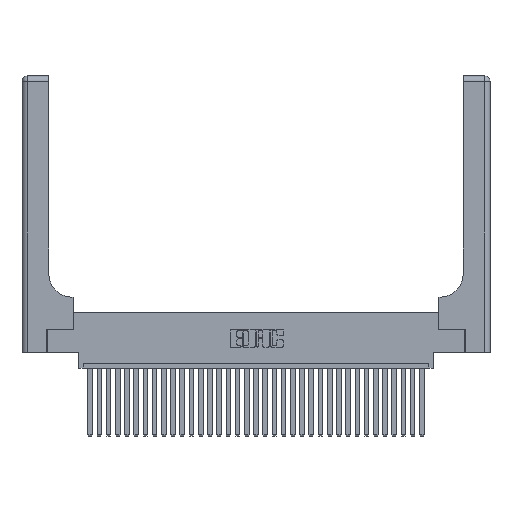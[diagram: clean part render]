
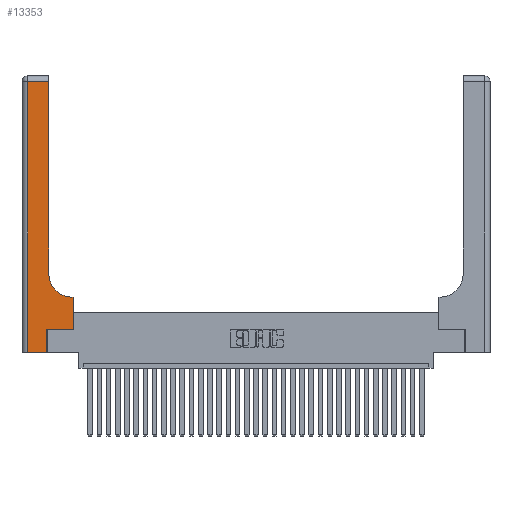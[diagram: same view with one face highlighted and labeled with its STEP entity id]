
A CAD part, top view. The second image highlights one B-rep face of the part: STEP entity #13353.
In plain terms, the highlighted planar face has unit normal (0, 0, 1).
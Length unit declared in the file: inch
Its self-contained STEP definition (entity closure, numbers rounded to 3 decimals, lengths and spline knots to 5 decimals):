
#236 = VERTEX_POINT ( 'NONE', #25386 ) ;
#242 = CARTESIAN_POINT ( 'NONE',  ( 0., 2.94, 0.37 ) ) ;
#461 = CARTESIAN_POINT ( 'NONE',  ( 0.269, 0.25, 0.37 ) ) ;
#1861 = VECTOR ( 'NONE', #8779, 39.37008 ) ;
#2887 = ORIENTED_EDGE ( 'NONE', *, *, #11937, .T. ) ;
#3539 = CARTESIAN_POINT ( 'NONE',  ( 0.2915, 3., 0.37 ) ) ;
#4384 = VERTEX_POINT ( 'NONE', #17243 ) ;
#4516 = DIRECTION ( 'NONE',  ( -1., 0., 0. ) ) ;
#4655 = ORIENTED_EDGE ( 'NONE', *, *, #23702, .T. ) ;
#5035 = LINE ( 'NONE', #22407, #10288 ) ;
#6044 = LINE ( 'NONE', #19729, #22750 ) ;
#6705 = EDGE_CURVE ( 'NONE', #28600, #26477, #22042, .T. ) ;
#6734 = ORIENTED_EDGE ( 'NONE', *, *, #29484, .T. ) ;
#7010 = ORIENTED_EDGE ( 'NONE', *, *, #10137, .T. ) ;
#7316 = CARTESIAN_POINT ( 'NONE',  ( 0., 0., 0.37 ) ) ;
#8605 = VERTEX_POINT ( 'NONE', #30904 ) ;
#8779 = DIRECTION ( 'NONE',  ( 1., 0., 0. ) ) ;
#9307 = VERTEX_POINT ( 'NONE', #14471 ) ;
#9494 = PLANE ( 'NONE',  #14238 ) ;
#9602 = CARTESIAN_POINT ( 'NONE',  ( 0.2915, 0.85, 0.37 ) ) ;
#10137 = EDGE_CURVE ( 'NONE', #236, #22982, #5035, .T. ) ;
#10195 = AXIS2_PLACEMENT_3D ( 'NONE', #28456, #26168, #23235 ) ;
#10288 = VECTOR ( 'NONE', #32861, 39.37008 ) ;
#10677 = ORIENTED_EDGE ( 'NONE', *, *, #17491, .T. ) ;
#11116 = CARTESIAN_POINT ( 'NONE',  ( 0.269, 0.25, 0.37 ) ) ;
#11161 = VERTEX_POINT ( 'NONE', #17155 ) ;
#11925 = LINE ( 'NONE', #7316, #25725 ) ;
#11937 = EDGE_CURVE ( 'NONE', #26477, #236, #14668, .T. ) ;
#12124 = EDGE_CURVE ( 'NONE', #9307, #11161, #22380, .T. ) ;
#12265 = CARTESIAN_POINT ( 'NONE',  ( 0.2915, 0.6, 0.37 ) ) ;
#13136 = VECTOR ( 'NONE', #26936, 39.37008 ) ;
#13353 = ADVANCED_FACE ( 'NONE', ( #23952 ), #9494, .F. ) ;
#13553 = EDGE_CURVE ( 'NONE', #8605, #17045, #6044, .T. ) ;
#14238 = AXIS2_PLACEMENT_3D ( 'NONE', #20008, #14987, #33146 ) ;
#14471 = CARTESIAN_POINT ( 'NONE',  ( 0.5585, 0.25, 0.37 ) ) ;
#14668 = LINE ( 'NONE', #242, #19956 ) ;
#14987 = DIRECTION ( 'NONE',  ( 0., 0., -1. ) ) ;
#15759 = EDGE_LOOP ( 'NONE', ( #32564, #2887, #7010, #33232, #20125, #4655, #28439, #10677, #6734 ) ) ;
#15950 = CIRCLE ( 'NONE', #10195, 0.25 ) ;
#16035 = CARTESIAN_POINT ( 'NONE',  ( 0.06, 0., 0.37 ) ) ;
#17045 = VERTEX_POINT ( 'NONE', #461 ) ;
#17155 = CARTESIAN_POINT ( 'NONE',  ( 0.5585, 0.6, 0.37 ) ) ;
#17243 = CARTESIAN_POINT ( 'NONE',  ( 0.5415, 0.6, 0.37 ) ) ;
#17491 = EDGE_CURVE ( 'NONE', #11161, #4384, #28395, .T. ) ;
#19360 = LINE ( 'NONE', #11116, #1861 ) ;
#19667 = CARTESIAN_POINT ( 'NONE',  ( 0.5585, 0.25, 0.37 ) ) ;
#19729 = CARTESIAN_POINT ( 'NONE',  ( 0.269, 0., 0.37 ) ) ;
#19956 = VECTOR ( 'NONE', #31246, 39.37008 ) ;
#20008 = CARTESIAN_POINT ( 'NONE',  ( 0., 3., 0.37 ) ) ;
#20125 = ORIENTED_EDGE ( 'NONE', *, *, #13553, .T. ) ;
#21134 = VECTOR ( 'NONE', #24529, 39.37008 ) ;
#21873 = VECTOR ( 'NONE', #4516, 39.37008 ) ;
#22042 = LINE ( 'NONE', #3539, #13136 ) ;
#22380 = LINE ( 'NONE', #19667, #21134 ) ;
#22407 = CARTESIAN_POINT ( 'NONE',  ( 0.06, 3., 0.37 ) ) ;
#22750 = VECTOR ( 'NONE', #33322, 39.37008 ) ;
#22982 = VERTEX_POINT ( 'NONE', #16035 ) ;
#23235 = DIRECTION ( 'NONE',  ( 1., 0., 0. ) ) ;
#23702 = EDGE_CURVE ( 'NONE', #17045, #9307, #19360, .T. ) ;
#23952 = FACE_OUTER_BOUND ( 'NONE', #15759, .T. ) ;
#24529 = DIRECTION ( 'NONE',  ( 0., 1., 0. ) ) ;
#25386 = CARTESIAN_POINT ( 'NONE',  ( 0.06, 2.94, 0.37 ) ) ;
#25646 = EDGE_CURVE ( 'NONE', #22982, #8605, #11925, .T. ) ;
#25725 = VECTOR ( 'NONE', #25759, 39.37008 ) ;
#25759 = DIRECTION ( 'NONE',  ( 1., 0., 0. ) ) ;
#26168 = DIRECTION ( 'NONE',  ( 0., 0., -1. ) ) ;
#26477 = VERTEX_POINT ( 'NONE', #29127 ) ;
#26936 = DIRECTION ( 'NONE',  ( 0., 1., 0. ) ) ;
#28395 = LINE ( 'NONE', #12265, #21873 ) ;
#28439 = ORIENTED_EDGE ( 'NONE', *, *, #12124, .T. ) ;
#28456 = CARTESIAN_POINT ( 'NONE',  ( 0.5415, 0.85, 0.37 ) ) ;
#28600 = VERTEX_POINT ( 'NONE', #9602 ) ;
#29127 = CARTESIAN_POINT ( 'NONE',  ( 0.2915, 2.94, 0.37 ) ) ;
#29484 = EDGE_CURVE ( 'NONE', #4384, #28600, #15950, .T. ) ;
#30904 = CARTESIAN_POINT ( 'NONE',  ( 0.269, 0., 0.37 ) ) ;
#31246 = DIRECTION ( 'NONE',  ( -1., 0., 0. ) ) ;
#32564 = ORIENTED_EDGE ( 'NONE', *, *, #6705, .T. ) ;
#32861 = DIRECTION ( 'NONE',  ( 0., -1., 0. ) ) ;
#33146 = DIRECTION ( 'NONE',  ( -1., 0., 0. ) ) ;
#33232 = ORIENTED_EDGE ( 'NONE', *, *, #25646, .T. ) ;
#33322 = DIRECTION ( 'NONE',  ( 0., 1., 0. ) ) ;
